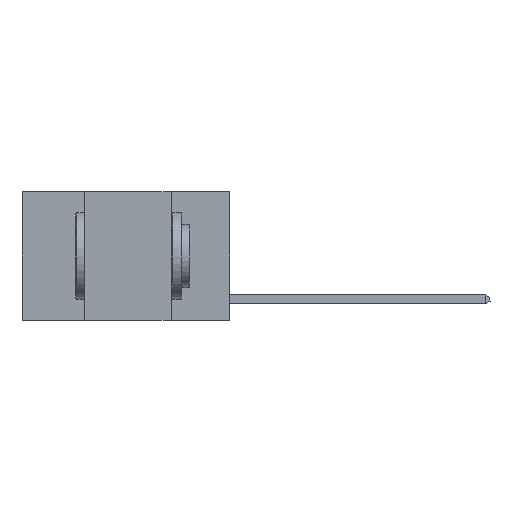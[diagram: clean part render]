
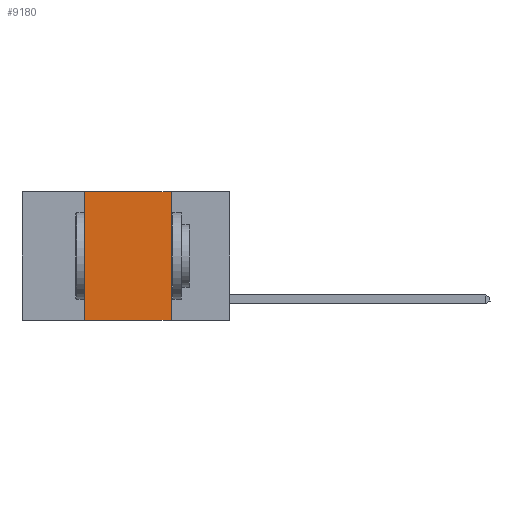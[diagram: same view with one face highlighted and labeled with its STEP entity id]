
A CAD part, left-side view. The second image highlights one B-rep face of the part: STEP entity #9180.
In plain terms, the highlighted planar face has unit normal (-1, 0, 0).
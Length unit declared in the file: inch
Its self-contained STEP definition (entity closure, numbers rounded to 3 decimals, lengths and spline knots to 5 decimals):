
#22 = EDGE_CURVE ( 'NONE', #1873, #10631, #6492, .T. ) ;
#948 = DIRECTION ( 'NONE',  ( 0., 0., -1. ) ) ;
#965 = EDGE_LOOP ( 'NONE', ( #1987, #3997, #4826, #4969 ) ) ;
#1509 = EDGE_CURVE ( 'NONE', #9559, #2610, #5435, .T. ) ;
#1514 = DIRECTION ( 'NONE',  ( 0., -1., 0. ) ) ;
#1533 = VECTOR ( 'NONE', #6784, 39.37008 ) ;
#1873 = VERTEX_POINT ( 'NONE', #10325 ) ;
#1987 = ORIENTED_EDGE ( 'NONE', *, *, #4082, .F. ) ;
#2189 = PLANE ( 'NONE',  #11663 ) ;
#2610 = VERTEX_POINT ( 'NONE', #12427 ) ;
#3578 = CARTESIAN_POINT ( 'NONE',  ( 0., 0.17, 0. ) ) ;
#3997 = ORIENTED_EDGE ( 'NONE', *, *, #22, .F. ) ;
#4082 = EDGE_CURVE ( 'NONE', #10631, #2610, #12038, .T. ) ;
#4826 = ORIENTED_EDGE ( 'NONE', *, *, #7859, .F. ) ;
#4969 = ORIENTED_EDGE ( 'NONE', *, *, #1509, .T. ) ;
#5435 = LINE ( 'NONE', #6850, #1533 ) ;
#6492 = LINE ( 'NONE', #9166, #9920 ) ;
#6784 = DIRECTION ( 'NONE',  ( 0., -1., 0. ) ) ;
#6850 = CARTESIAN_POINT ( 'NONE',  ( 0., 0.6, -0.37 ) ) ;
#7737 = DIRECTION ( 'NONE',  ( 0., 0., -1. ) ) ;
#7859 = EDGE_CURVE ( 'NONE', #9559, #1873, #10284, .T. ) ;
#8538 = VECTOR ( 'NONE', #7737, 39.37008 ) ;
#8681 = DIRECTION ( 'NONE',  ( 1., 0., 0. ) ) ;
#9166 = CARTESIAN_POINT ( 'NONE',  ( 0., 0.6, 0. ) ) ;
#9180 = ADVANCED_FACE ( 'NONE', ( #13755 ), #2189, .F. ) ;
#9559 = VERTEX_POINT ( 'NONE', #10767 ) ;
#9861 = VECTOR ( 'NONE', #15479, 39.37008 ) ;
#9920 = VECTOR ( 'NONE', #1514, 39.37008 ) ;
#10284 = LINE ( 'NONE', #14271, #9861 ) ;
#10325 = CARTESIAN_POINT ( 'NONE',  ( 0., 0.42, 0. ) ) ;
#10631 = VERTEX_POINT ( 'NONE', #3578 ) ;
#10767 = CARTESIAN_POINT ( 'NONE',  ( 0., 0.42, -0.37 ) ) ;
#11663 = AXIS2_PLACEMENT_3D ( 'NONE', #13856, #8681, #948 ) ;
#12038 = LINE ( 'NONE', #15406, #8538 ) ;
#12427 = CARTESIAN_POINT ( 'NONE',  ( 0., 0.17, -0.37 ) ) ;
#13755 = FACE_OUTER_BOUND ( 'NONE', #965, .T. ) ;
#13856 = CARTESIAN_POINT ( 'NONE',  ( 0., 0.6, 0. ) ) ;
#14271 = CARTESIAN_POINT ( 'NONE',  ( 0., 0.42, 0. ) ) ;
#15406 = CARTESIAN_POINT ( 'NONE',  ( 0., 0.17, 0. ) ) ;
#15479 = DIRECTION ( 'NONE',  ( 0., 0., 1. ) ) ;
